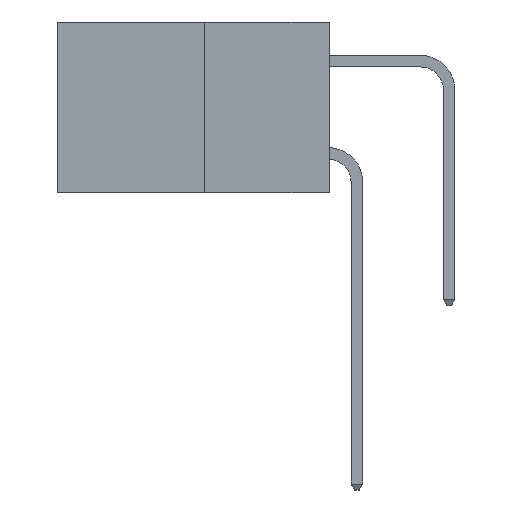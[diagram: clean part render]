
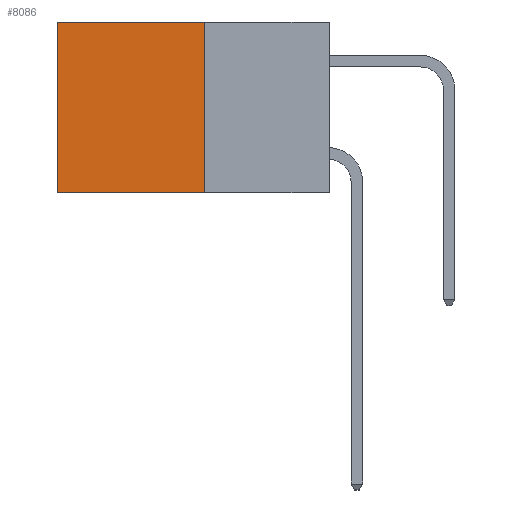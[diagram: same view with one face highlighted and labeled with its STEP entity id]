
A CAD part, left-side view. The second image highlights one B-rep face of the part: STEP entity #8086.
In plain terms, the highlighted planar face has unit normal (-1, 0, 0).
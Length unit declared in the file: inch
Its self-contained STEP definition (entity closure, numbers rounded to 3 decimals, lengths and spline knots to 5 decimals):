
#493 = DIRECTION ( 'NONE',  ( 0., 0., -1. ) ) ;
#808 = DIRECTION ( 'NONE',  ( 0., 1., 0. ) ) ;
#2782 = LINE ( 'NONE', #16649, #14775 ) ;
#2873 = ORIENTED_EDGE ( 'NONE', *, *, #16046, .T. ) ;
#2879 = DIRECTION ( 'NONE',  ( 0., 0., -1. ) ) ;
#2930 = AXIS2_PLACEMENT_3D ( 'NONE', #3410, #3026, #2879 ) ;
#3026 = DIRECTION ( 'NONE',  ( 1., 0., 0. ) ) ;
#3410 = CARTESIAN_POINT ( 'NONE',  ( 0.277, 0.27, -0.37 ) ) ;
#3511 = CARTESIAN_POINT ( 'NONE',  ( 0.277, 0.59, 0. ) ) ;
#3646 = EDGE_CURVE ( 'NONE', #12651, #9774, #11615, .T. ) ;
#3657 = PLANE ( 'NONE',  #2930 ) ;
#4930 = ORIENTED_EDGE ( 'NONE', *, *, #15602, .T. ) ;
#5081 = CARTESIAN_POINT ( 'NONE',  ( 0.277, 0.27, 0. ) ) ;
#5689 = EDGE_LOOP ( 'NONE', ( #4930, #10087, #8726, #2873 ) ) ;
#5821 = FACE_OUTER_BOUND ( 'NONE', #5689, .T. ) ;
#6354 = VECTOR ( 'NONE', #6666, 39.37008 ) ;
#6440 = CARTESIAN_POINT ( 'NONE',  ( 0.277, 0.27, 0. ) ) ;
#6666 = DIRECTION ( 'NONE',  ( 0., 1., 0. ) ) ;
#6828 = LINE ( 'NONE', #11704, #10981 ) ;
#7233 = DIRECTION ( 'NONE',  ( 0., 0., -1. ) ) ;
#7455 = VECTOR ( 'NONE', #493, 39.37008 ) ;
#7530 = CARTESIAN_POINT ( 'NONE',  ( 0.277, 0.59, -0.37 ) ) ;
#8086 = ADVANCED_FACE ( 'NONE', ( #5821 ), #3657, .F. ) ;
#8726 = ORIENTED_EDGE ( 'NONE', *, *, #3646, .F. ) ;
#9774 = VERTEX_POINT ( 'NONE', #13036 ) ;
#10087 = ORIENTED_EDGE ( 'NONE', *, *, #16892, .F. ) ;
#10981 = VECTOR ( 'NONE', #808, 39.37008 ) ;
#11615 = LINE ( 'NONE', #17043, #7455 ) ;
#11704 = CARTESIAN_POINT ( 'NONE',  ( 0.277, 0.27, -0.37 ) ) ;
#12651 = VERTEX_POINT ( 'NONE', #6440 ) ;
#13036 = CARTESIAN_POINT ( 'NONE',  ( 0.277, 0.27, -0.37 ) ) ;
#14775 = VECTOR ( 'NONE', #7233, 39.37008 ) ;
#15602 = EDGE_CURVE ( 'NONE', #19920, #17116, #2782, .T. ) ;
#16046 = EDGE_CURVE ( 'NONE', #12651, #19920, #19270, .T. ) ;
#16649 = CARTESIAN_POINT ( 'NONE',  ( 0.277, 0.59, -0.37 ) ) ;
#16892 = EDGE_CURVE ( 'NONE', #9774, #17116, #6828, .T. ) ;
#17043 = CARTESIAN_POINT ( 'NONE',  ( 0.277, 0.27, -0.37 ) ) ;
#17116 = VERTEX_POINT ( 'NONE', #7530 ) ;
#19270 = LINE ( 'NONE', #5081, #6354 ) ;
#19920 = VERTEX_POINT ( 'NONE', #3511 ) ;
